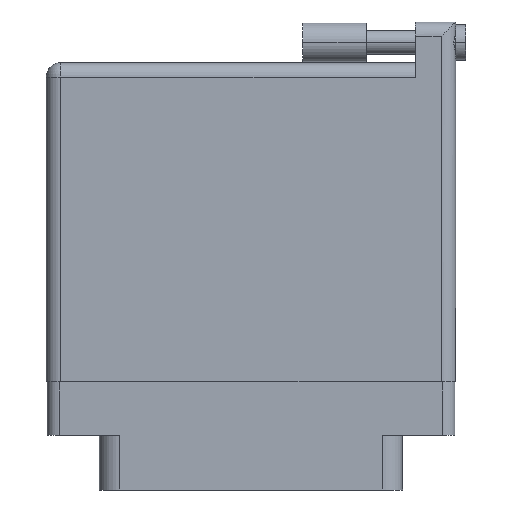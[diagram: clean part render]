
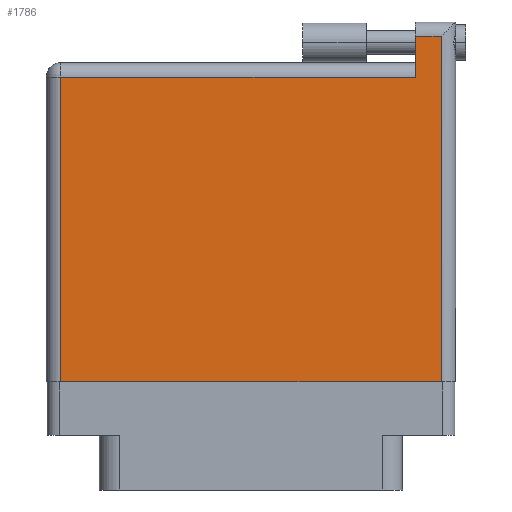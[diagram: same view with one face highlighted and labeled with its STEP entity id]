
A CAD part, front view. The second image highlights one B-rep face of the part: STEP entity #1786.
In plain terms, the highlighted face is planar.
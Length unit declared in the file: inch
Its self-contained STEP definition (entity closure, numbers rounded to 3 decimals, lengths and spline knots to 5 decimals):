
#176 = LINE ( 'NONE', #19565, #22349 ) ;
#266 = DIRECTION ( 'NONE',  ( -1., 0., 0. ) ) ;
#836 = VECTOR ( 'NONE', #266, 39.37008 ) ;
#1045 = EDGE_LOOP ( 'NONE', ( #22332, #4526, #21521, #5042, #2861, #15352 ) ) ;
#1238 = LINE ( 'NONE', #5072, #30547 ) ;
#1455 = CARTESIAN_POINT ( 'NONE',  ( 1.811, 1.766, 0. ) ) ;
#1786 = ADVANCED_FACE ( 'NONE', ( #32464 ), #31841, .F. ) ;
#2033 = VERTEX_POINT ( 'NONE', #11910 ) ;
#2861 = ORIENTED_EDGE ( 'NONE', *, *, #34724, .T. ) ;
#4364 = EDGE_CURVE ( 'NONE', #6858, #21640, #1238, .T. ) ;
#4526 = ORIENTED_EDGE ( 'NONE', *, *, #16298, .T. ) ;
#4790 = CARTESIAN_POINT ( 'NONE',  ( 1.938, 0., 0. ) ) ;
#5042 = ORIENTED_EDGE ( 'NONE', *, *, #25358, .T. ) ;
#5072 = CARTESIAN_POINT ( 'NONE',  ( 0., 0., 0. ) ) ;
#6090 = CARTESIAN_POINT ( 'NONE',  ( 1.938, 1.696, 0. ) ) ;
#6858 = VERTEX_POINT ( 'NONE', #28298 ) ;
#7518 = DIRECTION ( 'NONE',  ( 0., -1., 0. ) ) ;
#7711 = CARTESIAN_POINT ( 'NONE',  ( 0., 1.566, 0. ) ) ;
#8046 = CARTESIAN_POINT ( 'NONE',  ( 1.811, 1.696, 0. ) ) ;
#8221 = CARTESIAN_POINT ( 'NONE',  ( 0., 1.696, 0. ) ) ;
#10646 = DIRECTION ( 'NONE',  ( -1., 0., 0. ) ) ;
#11625 = DIRECTION ( 'NONE',  ( -1., 0., 0. ) ) ;
#11910 = CARTESIAN_POINT ( 'NONE',  ( 0.07, 1.496, 0. ) ) ;
#12781 = DIRECTION ( 'NONE',  ( 0., 1., 0. ) ) ;
#13286 = DIRECTION ( 'NONE',  ( 1., 0., 0. ) ) ;
#15352 = ORIENTED_EDGE ( 'NONE', *, *, #27034, .T. ) ;
#15482 = LINE ( 'NONE', #23902, #17152 ) ;
#15825 = LINE ( 'NONE', #23884, #34280 ) ;
#16298 = EDGE_CURVE ( 'NONE', #21640, #30212, #15825, .T. ) ;
#16631 = VERTEX_POINT ( 'NONE', #27369 ) ;
#17152 = VECTOR ( 'NONE', #7518, 39.37008 ) ;
#19378 = VECTOR ( 'NONE', #20264, 39.37008 ) ;
#19565 = CARTESIAN_POINT ( 'NONE',  ( 0., 1.496, 0. ) ) ;
#20264 = DIRECTION ( 'NONE',  ( 0., -1., 0. ) ) ;
#21521 = ORIENTED_EDGE ( 'NONE', *, *, #31971, .T. ) ;
#21640 = VERTEX_POINT ( 'NONE', #4790 ) ;
#22332 = ORIENTED_EDGE ( 'NONE', *, *, #4364, .T. ) ;
#22349 = VECTOR ( 'NONE', #11625, 39.37008 ) ;
#23421 = LINE ( 'NONE', #8221, #836 ) ;
#23884 = CARTESIAN_POINT ( 'NONE',  ( 1.938, 1.766, 0. ) ) ;
#23902 = CARTESIAN_POINT ( 'NONE',  ( 0.07, 0., 0. ) ) ;
#24811 = LINE ( 'NONE', #1455, #19378 ) ;
#25358 = EDGE_CURVE ( 'NONE', #28566, #16631, #24811, .T. ) ;
#27034 = EDGE_CURVE ( 'NONE', #2033, #6858, #15482, .T. ) ;
#27369 = CARTESIAN_POINT ( 'NONE',  ( 1.811, 1.496, 0. ) ) ;
#28298 = CARTESIAN_POINT ( 'NONE',  ( 0.07, 0., 0. ) ) ;
#28566 = VERTEX_POINT ( 'NONE', #8046 ) ;
#29058 = AXIS2_PLACEMENT_3D ( 'NONE', #7711, #29226, #10646 ) ;
#29226 = DIRECTION ( 'NONE',  ( 0., 0., -1. ) ) ;
#30212 = VERTEX_POINT ( 'NONE', #6090 ) ;
#30547 = VECTOR ( 'NONE', #13286, 39.37008 ) ;
#31841 = PLANE ( 'NONE',  #29058 ) ;
#31971 = EDGE_CURVE ( 'NONE', #30212, #28566, #23421, .T. ) ;
#32464 = FACE_OUTER_BOUND ( 'NONE', #1045, .T. ) ;
#34280 = VECTOR ( 'NONE', #12781, 39.37008 ) ;
#34724 = EDGE_CURVE ( 'NONE', #16631, #2033, #176, .T. ) ;
